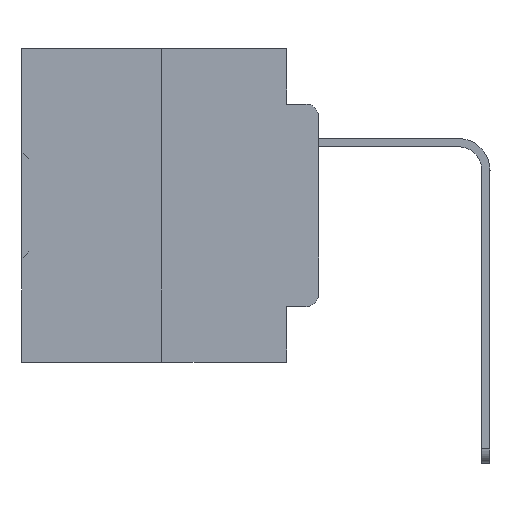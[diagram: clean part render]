
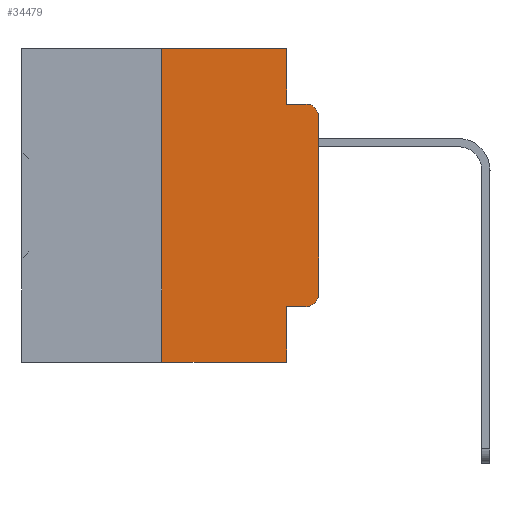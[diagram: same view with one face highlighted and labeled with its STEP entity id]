
A CAD part, left-side view. The second image highlights one B-rep face of the part: STEP entity #34479.
In plain terms, the highlighted planar face has unit normal (-1, 0, 0).
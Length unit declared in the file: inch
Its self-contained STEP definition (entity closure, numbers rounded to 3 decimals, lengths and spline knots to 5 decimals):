
#581 = ORIENTED_EDGE ( 'NONE', *, *, #22406, .F. ) ;
#591 = ORIENTED_EDGE ( 'NONE', *, *, #12841, .T. ) ;
#1414 = VERTEX_POINT ( 'NONE', #6634 ) ;
#1942 = CARTESIAN_POINT ( 'NONE',  ( 0., 0.051, -0.0885 ) ) ;
#1953 = CARTESIAN_POINT ( 'NONE',  ( 0., 0.051, 0. ) ) ;
#1974 = ORIENTED_EDGE ( 'NONE', *, *, #14003, .T. ) ;
#2578 = CARTESIAN_POINT ( 'NONE',  ( 0., 0.051, -0.5 ) ) ;
#3661 = DIRECTION ( 'NONE',  ( 0., -1., 0. ) ) ;
#3863 = VECTOR ( 'NONE', #25263, 39.37008 ) ;
#4109 = VERTEX_POINT ( 'NONE', #26956 ) ;
#4536 = CARTESIAN_POINT ( 'NONE',  ( 0., 0.02, -0.1085 ) ) ;
#5216 = AXIS2_PLACEMENT_3D ( 'NONE', #12081, #34005, #28610 ) ;
#5479 = VECTOR ( 'NONE', #26056, 39.37008 ) ;
#6583 = VECTOR ( 'NONE', #36024, 39.37008 ) ;
#6634 = CARTESIAN_POINT ( 'NONE',  ( 0., 0.02, -0.0885 ) ) ;
#6885 = VERTEX_POINT ( 'NONE', #32136 ) ;
#7340 = DIRECTION ( 'NONE',  ( 0., 0., -1. ) ) ;
#7712 = EDGE_CURVE ( 'NONE', #12389, #25753, #33491, .T. ) ;
#7830 = EDGE_CURVE ( 'NONE', #4109, #18279, #14273, .T. ) ;
#8207 = EDGE_LOOP ( 'NONE', ( #13956, #591, #25284, #29565, #25352, #581, #35746, #31798, #1974, #17780 ) ) ;
#9034 = PLANE ( 'NONE',  #5216 ) ;
#11837 = VERTEX_POINT ( 'NONE', #22364 ) ;
#12081 = CARTESIAN_POINT ( 'NONE',  ( 0., 0.473, 0. ) ) ;
#12388 = VECTOR ( 'NONE', #34263, 39.37008 ) ;
#12389 = VERTEX_POINT ( 'NONE', #24288 ) ;
#12580 = VERTEX_POINT ( 'NONE', #14767 ) ;
#12753 = VECTOR ( 'NONE', #3661, 39.37008 ) ;
#12841 = EDGE_CURVE ( 'NONE', #34021, #1414, #31118, .T. ) ;
#13236 = LINE ( 'NONE', #30105, #27139 ) ;
#13956 = ORIENTED_EDGE ( 'NONE', *, *, #30846, .T. ) ;
#14003 = EDGE_CURVE ( 'NONE', #11837, #4109, #13236, .T. ) ;
#14273 = CIRCLE ( 'NONE', #34441, 0.02 ) ;
#14767 = CARTESIAN_POINT ( 'NONE',  ( 0., 0.051, 0. ) ) ;
#15537 = CARTESIAN_POINT ( 'NONE',  ( 0., 0.25, 0. ) ) ;
#17145 = LINE ( 'NONE', #34501, #12388 ) ;
#17579 = CARTESIAN_POINT ( 'NONE',  ( 0., 0., -0.1085 ) ) ;
#17780 = ORIENTED_EDGE ( 'NONE', *, *, #7830, .T. ) ;
#17970 = LINE ( 'NONE', #34354, #12753 ) ;
#18279 = VERTEX_POINT ( 'NONE', #28267 ) ;
#18498 = FACE_OUTER_BOUND ( 'NONE', #8207, .T. ) ;
#18795 = VECTOR ( 'NONE', #32364, 39.37008 ) ;
#20022 = CARTESIAN_POINT ( 'NONE',  ( 0., 0.02, -0.3915 ) ) ;
#20349 = CARTESIAN_POINT ( 'NONE',  ( 0., 0.051, 0. ) ) ;
#21368 = VERTEX_POINT ( 'NONE', #1942 ) ;
#21617 = DIRECTION ( 'NONE',  ( 0., -1., 0. ) ) ;
#22364 = CARTESIAN_POINT ( 'NONE',  ( 0., 0.051, -0.4115 ) ) ;
#22406 = EDGE_CURVE ( 'NONE', #12389, #6885, #25756, .T. ) ;
#22966 = EDGE_CURVE ( 'NONE', #12580, #21368, #27561, .T. ) ;
#24288 = CARTESIAN_POINT ( 'NONE',  ( 0., 0.25, -0.5 ) ) ;
#25263 = DIRECTION ( 'NONE',  ( 0., -1., 0. ) ) ;
#25284 = ORIENTED_EDGE ( 'NONE', *, *, #32467, .F. ) ;
#25352 = ORIENTED_EDGE ( 'NONE', *, *, #36000, .F. ) ;
#25753 = VERTEX_POINT ( 'NONE', #2578 ) ;
#25756 = LINE ( 'NONE', #15537, #18795 ) ;
#25923 = LINE ( 'NONE', #20349, #5479 ) ;
#26056 = DIRECTION ( 'NONE',  ( 0., 0., -1. ) ) ;
#26956 = CARTESIAN_POINT ( 'NONE',  ( 0., 0.02, -0.4115 ) ) ;
#27139 = VECTOR ( 'NONE', #21617, 39.37008 ) ;
#27329 = CARTESIAN_POINT ( 'NONE',  ( 0., 0.051, -0.0885 ) ) ;
#27561 = LINE ( 'NONE', #1953, #33254 ) ;
#27808 = CARTESIAN_POINT ( 'NONE',  ( 0., 0.473, -0.5 ) ) ;
#28267 = CARTESIAN_POINT ( 'NONE',  ( 0., 0., -0.3915 ) ) ;
#28610 = DIRECTION ( 'NONE',  ( 0., 0., -1. ) ) ;
#28653 = DIRECTION ( 'NONE',  ( -1., 0., 0. ) ) ;
#28895 = AXIS2_PLACEMENT_3D ( 'NONE', #4536, #35343, #7340 ) ;
#29565 = ORIENTED_EDGE ( 'NONE', *, *, #22966, .F. ) ;
#30105 = CARTESIAN_POINT ( 'NONE',  ( 0., 0.051, -0.4115 ) ) ;
#30514 = LINE ( 'NONE', #27329, #6583 ) ;
#30846 = EDGE_CURVE ( 'NONE', #18279, #34021, #17145, .T. ) ;
#31118 = CIRCLE ( 'NONE', #28895, 0.02 ) ;
#31442 = DIRECTION ( 'NONE',  ( 0., 0., -1. ) ) ;
#31798 = ORIENTED_EDGE ( 'NONE', *, *, #33419, .F. ) ;
#32136 = CARTESIAN_POINT ( 'NONE',  ( 0., 0.25, 0. ) ) ;
#32364 = DIRECTION ( 'NONE',  ( 0., 0., 1. ) ) ;
#32467 = EDGE_CURVE ( 'NONE', #21368, #1414, #30514, .T. ) ;
#33254 = VECTOR ( 'NONE', #35212, 39.37008 ) ;
#33419 = EDGE_CURVE ( 'NONE', #11837, #25753, #25923, .T. ) ;
#33491 = LINE ( 'NONE', #27808, #3863 ) ;
#34005 = DIRECTION ( 'NONE',  ( 1., 0., 0. ) ) ;
#34021 = VERTEX_POINT ( 'NONE', #17579 ) ;
#34263 = DIRECTION ( 'NONE',  ( 0., 0., 1. ) ) ;
#34354 = CARTESIAN_POINT ( 'NONE',  ( 0., 0.473, 0. ) ) ;
#34441 = AXIS2_PLACEMENT_3D ( 'NONE', #20022, #28653, #31442 ) ;
#34479 = ADVANCED_FACE ( 'NONE', ( #18498 ), #9034, .F. ) ;
#34501 = CARTESIAN_POINT ( 'NONE',  ( 0., 0., 0. ) ) ;
#35212 = DIRECTION ( 'NONE',  ( 0., 0., -1. ) ) ;
#35343 = DIRECTION ( 'NONE',  ( -1., 0., 0. ) ) ;
#35746 = ORIENTED_EDGE ( 'NONE', *, *, #7712, .T. ) ;
#36000 = EDGE_CURVE ( 'NONE', #6885, #12580, #17970, .T. ) ;
#36024 = DIRECTION ( 'NONE',  ( 0., -1., 0. ) ) ;
